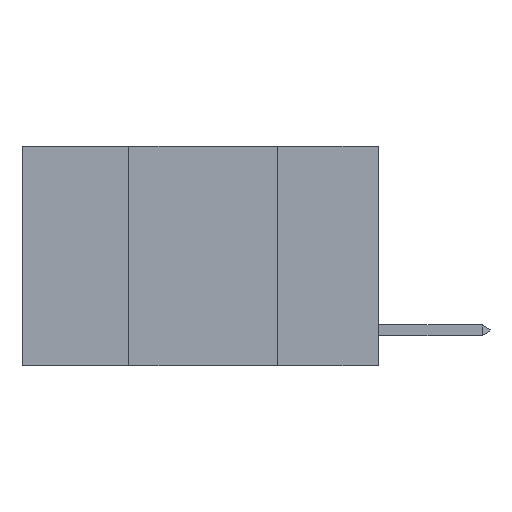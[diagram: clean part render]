
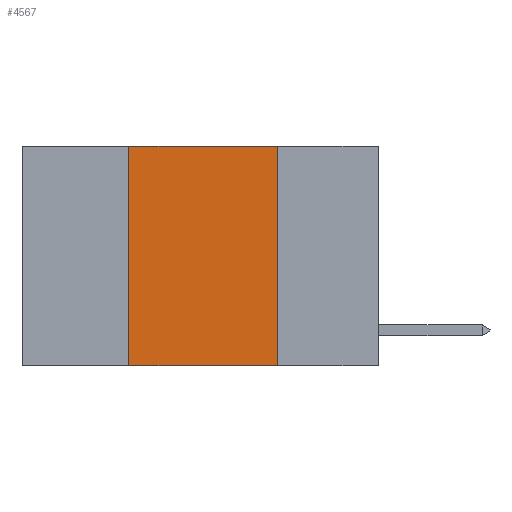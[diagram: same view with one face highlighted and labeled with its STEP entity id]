
A CAD part, left-side view. The second image highlights one B-rep face of the part: STEP entity #4567.
In plain terms, the highlighted planar face has unit normal (-1, 0, 0).
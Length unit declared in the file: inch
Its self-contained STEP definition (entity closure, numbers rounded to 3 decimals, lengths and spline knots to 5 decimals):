
#7 = AXIS2_PLACEMENT_3D ( 'NONE', #5685, #2784, #12242 ) ;
#866 = EDGE_CURVE ( 'NONE', #12674, #8737, #10897, .T. ) ;
#958 = EDGE_CURVE ( 'NONE', #8737, #15337, #18118, .T. ) ;
#1134 = VECTOR ( 'NONE', #19661, 39.37008 ) ;
#1527 = VECTOR ( 'NONE', #11285, 39.37008 ) ;
#2241 = VERTEX_POINT ( 'NONE', #6186 ) ;
#2692 = ORIENTED_EDGE ( 'NONE', *, *, #10286, .T. ) ;
#2784 = DIRECTION ( 'NONE',  ( 1., 0., 0. ) ) ;
#2965 = DIRECTION ( 'NONE',  ( 0., -1., 0. ) ) ;
#4567 = ADVANCED_FACE ( 'NONE', ( #10930 ), #17506, .F. ) ;
#5598 = CARTESIAN_POINT ( 'NONE',  ( 0., 0.17, 0. ) ) ;
#5685 = CARTESIAN_POINT ( 'NONE',  ( 0., 0.6, 0. ) ) ;
#6186 = CARTESIAN_POINT ( 'NONE',  ( 0., 0.42, -0.37 ) ) ;
#7112 = ORIENTED_EDGE ( 'NONE', *, *, #866, .F. ) ;
#7885 = ORIENTED_EDGE ( 'NONE', *, *, #11995, .F. ) ;
#8493 = CARTESIAN_POINT ( 'NONE',  ( 0., 0.6, -0.37 ) ) ;
#8737 = VERTEX_POINT ( 'NONE', #5598 ) ;
#9934 = VECTOR ( 'NONE', #2965, 39.37008 ) ;
#10033 = CARTESIAN_POINT ( 'NONE',  ( 0., 0.17, 0. ) ) ;
#10286 = EDGE_CURVE ( 'NONE', #2241, #15337, #16669, .T. ) ;
#10312 = VECTOR ( 'NONE', #16616, 39.37008 ) ;
#10777 = ORIENTED_EDGE ( 'NONE', *, *, #958, .F. ) ;
#10897 = LINE ( 'NONE', #12727, #9934 ) ;
#10930 = FACE_OUTER_BOUND ( 'NONE', #11601, .T. ) ;
#11285 = DIRECTION ( 'NONE',  ( 0., 0., 1. ) ) ;
#11601 = EDGE_LOOP ( 'NONE', ( #10777, #7112, #7885, #2692 ) ) ;
#11995 = EDGE_CURVE ( 'NONE', #2241, #12674, #14301, .T. ) ;
#12242 = DIRECTION ( 'NONE',  ( 0., 0., -1. ) ) ;
#12674 = VERTEX_POINT ( 'NONE', #18748 ) ;
#12727 = CARTESIAN_POINT ( 'NONE',  ( 0., 0.6, 0. ) ) ;
#14301 = LINE ( 'NONE', #20853, #1527 ) ;
#15337 = VERTEX_POINT ( 'NONE', #20486 ) ;
#16616 = DIRECTION ( 'NONE',  ( 0., 0., -1. ) ) ;
#16669 = LINE ( 'NONE', #8493, #1134 ) ;
#17506 = PLANE ( 'NONE',  #7 ) ;
#18118 = LINE ( 'NONE', #10033, #10312 ) ;
#18748 = CARTESIAN_POINT ( 'NONE',  ( 0., 0.42, 0. ) ) ;
#19661 = DIRECTION ( 'NONE',  ( 0., -1., 0. ) ) ;
#20486 = CARTESIAN_POINT ( 'NONE',  ( 0., 0.17, -0.37 ) ) ;
#20853 = CARTESIAN_POINT ( 'NONE',  ( 0., 0.42, 0. ) ) ;
